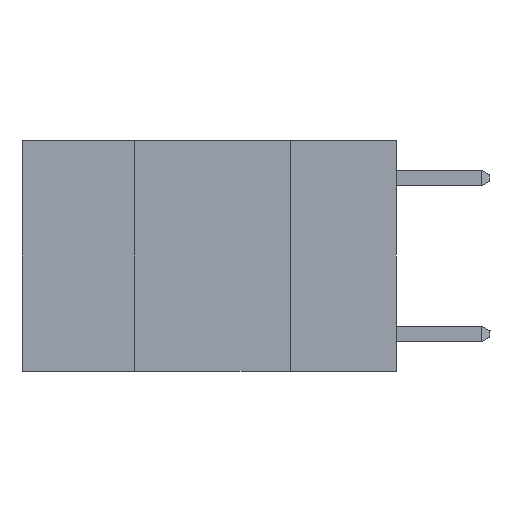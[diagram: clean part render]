
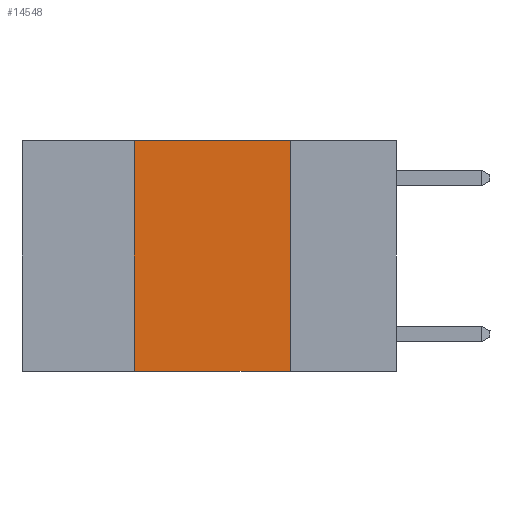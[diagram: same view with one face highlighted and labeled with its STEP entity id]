
A CAD part, left-side view. The second image highlights one B-rep face of the part: STEP entity #14548.
In plain terms, the highlighted planar face has unit normal (-1, 0, 0).
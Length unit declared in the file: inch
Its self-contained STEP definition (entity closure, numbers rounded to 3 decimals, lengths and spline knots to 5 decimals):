
#118 = CARTESIAN_POINT ( 'NONE',  ( 0., 0.17, 0. ) ) ;
#278 = DIRECTION ( 'NONE',  ( 1., 0., 0. ) ) ;
#753 = VECTOR ( 'NONE', #19373, 39.37008 ) ;
#1042 = AXIS2_PLACEMENT_3D ( 'NONE', #11482, #278, #13286 ) ;
#2128 = VECTOR ( 'NONE', #16779, 39.37008 ) ;
#3157 = LINE ( 'NONE', #12030, #12451 ) ;
#3945 = VERTEX_POINT ( 'NONE', #19733 ) ;
#4734 = ORIENTED_EDGE ( 'NONE', *, *, #9325, .F. ) ;
#5280 = ORIENTED_EDGE ( 'NONE', *, *, #14792, .F. ) ;
#5811 = LINE ( 'NONE', #15644, #753 ) ;
#5942 = PLANE ( 'NONE',  #1042 ) ;
#6390 = EDGE_LOOP ( 'NONE', ( #4734, #5280, #8424, #13927 ) ) ;
#6538 = CARTESIAN_POINT ( 'NONE',  ( 0., 0.17, -0.37 ) ) ;
#6855 = EDGE_CURVE ( 'NONE', #11276, #10850, #5811, .T. ) ;
#8080 = EDGE_CURVE ( 'NONE', #11276, #3945, #14028, .T. ) ;
#8424 = ORIENTED_EDGE ( 'NONE', *, *, #8080, .F. ) ;
#8712 = VERTEX_POINT ( 'NONE', #22289 ) ;
#9233 = VECTOR ( 'NONE', #17137, 39.37008 ) ;
#9325 = EDGE_CURVE ( 'NONE', #8712, #10850, #21572, .T. ) ;
#10850 = VERTEX_POINT ( 'NONE', #6538 ) ;
#11276 = VERTEX_POINT ( 'NONE', #15087 ) ;
#11482 = CARTESIAN_POINT ( 'NONE',  ( 0., 0.6, 0. ) ) ;
#12030 = CARTESIAN_POINT ( 'NONE',  ( 0., 0.6, 0. ) ) ;
#12451 = VECTOR ( 'NONE', #22707, 39.37008 ) ;
#13286 = DIRECTION ( 'NONE',  ( 0., 0., -1. ) ) ;
#13927 = ORIENTED_EDGE ( 'NONE', *, *, #6855, .T. ) ;
#14028 = LINE ( 'NONE', #22396, #9233 ) ;
#14548 = ADVANCED_FACE ( 'NONE', ( #16964 ), #5942, .F. ) ;
#14792 = EDGE_CURVE ( 'NONE', #3945, #8712, #3157, .T. ) ;
#15087 = CARTESIAN_POINT ( 'NONE',  ( 0., 0.42, -0.37 ) ) ;
#15644 = CARTESIAN_POINT ( 'NONE',  ( 0., 0.6, -0.37 ) ) ;
#16779 = DIRECTION ( 'NONE',  ( 0., 0., -1. ) ) ;
#16964 = FACE_OUTER_BOUND ( 'NONE', #6390, .T. ) ;
#17137 = DIRECTION ( 'NONE',  ( 0., 0., 1. ) ) ;
#19373 = DIRECTION ( 'NONE',  ( 0., -1., 0. ) ) ;
#19733 = CARTESIAN_POINT ( 'NONE',  ( 0., 0.42, 0. ) ) ;
#21572 = LINE ( 'NONE', #118, #2128 ) ;
#22289 = CARTESIAN_POINT ( 'NONE',  ( 0., 0.17, 0. ) ) ;
#22396 = CARTESIAN_POINT ( 'NONE',  ( 0., 0.42, 0. ) ) ;
#22707 = DIRECTION ( 'NONE',  ( 0., -1., 0. ) ) ;
